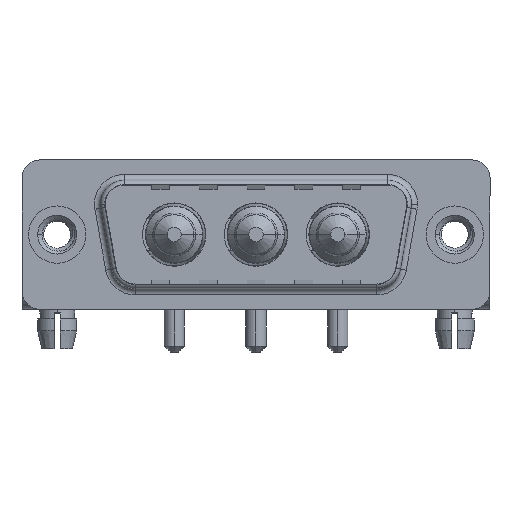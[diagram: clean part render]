
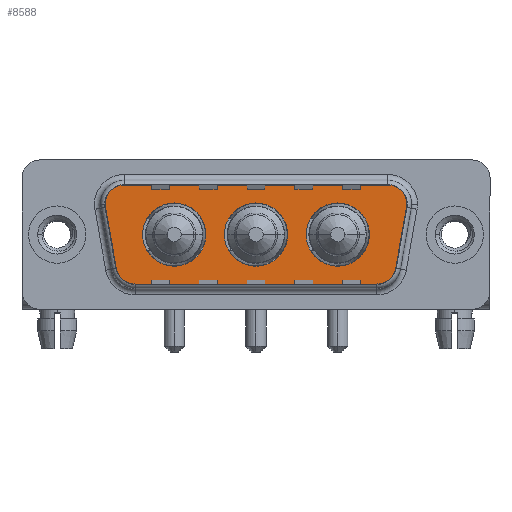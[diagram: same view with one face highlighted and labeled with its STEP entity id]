
A CAD part, top view. The second image highlights one B-rep face of the part: STEP entity #8588.
In plain terms, the highlighted planar face has unit normal (0, 0, 1).
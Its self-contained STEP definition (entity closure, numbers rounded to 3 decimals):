
#421 = ORIENTED_EDGE ( 'NONE', *, *, #2245, .F. ) ;
#662 = VERTEX_POINT ( 'NONE', #5880 ) ;
#727 = DIRECTION ( 'NONE',  ( 0.174, -0.985, 0. ) ) ;
#827 = DIRECTION ( 'NONE',  ( 0., 0., 1. ) ) ;
#843 = AXIS2_PLACEMENT_3D ( 'NONE', #4515, #4436, #9193 ) ;
#875 = EDGE_CURVE ( 'NONE', #9077, #4054, #5537, .T. ) ;
#971 = VECTOR ( 'NONE', #7393, 1000. ) ;
#1260 = CARTESIAN_POINT ( 'NONE',  ( 19.3, 0., 0. ) ) ;
#1284 = DIRECTION ( 'NONE',  ( 1., 0., 0. ) ) ;
#1347 = DIRECTION ( 'NONE',  ( 0., 0., 1. ) ) ;
#1507 = VECTOR ( 'NONE', #13732, 1000. ) ;
#1747 = VERTEX_POINT ( 'NONE', #15391 ) ;
#1857 = CARTESIAN_POINT ( 'NONE',  ( 26.866, -4.9, 0. ) ) ;
#1952 = ORIENTED_EDGE ( 'NONE', *, *, #10803, .F. ) ;
#2059 = CARTESIAN_POINT ( 'NONE',  ( 16.65, 0., 0. ) ) ;
#2143 = CARTESIAN_POINT ( 'NONE',  ( 3.441, 2.553, 0. ) ) ;
#2179 = AXIS2_PLACEMENT_3D ( 'NONE', #13234, #3705, #9710 ) ;
#2240 = CARTESIAN_POINT ( 'NONE',  ( 6.434, -4.9, 0. ) ) ;
#2245 = EDGE_CURVE ( 'NONE', #8454, #3330, #14317, .T. ) ;
#2381 = AXIS2_PLACEMENT_3D ( 'NONE', #6472, #11248, #10149 ) ;
#2434 = DIRECTION ( 'NONE',  ( 1., 0., 0. ) ) ;
#2448 = DIRECTION ( 'NONE',  ( 0., 0., 1. ) ) ;
#2454 = LINE ( 'NONE', #5647, #15405 ) ;
#2497 = EDGE_CURVE ( 'NONE', #8387, #662, #7977, .T. ) ;
#2549 = EDGE_CURVE ( 'NONE', #3667, #9077, #8069, .T. ) ;
#2558 = AXIS2_PLACEMENT_3D ( 'NONE', #6424, #7535, #4093 ) ;
#2796 = LINE ( 'NONE', #6372, #1507 ) ;
#2997 = VECTOR ( 'NONE', #727, 1000. ) ;
#3062 = EDGE_LOOP ( 'NONE', ( #7144, #14014, #3810, #6294, #6666, #3516, #14656, #10822, #7431 ) ) ;
#3122 = CARTESIAN_POINT ( 'NONE',  ( 29.859, 2.553, 0. ) ) ;
#3330 = VERTEX_POINT ( 'NONE', #1260 ) ;
#3516 = ORIENTED_EDGE ( 'NONE', *, *, #11779, .T. ) ;
#3667 = VERTEX_POINT ( 'NONE', #10840 ) ;
#3674 = CIRCLE ( 'NONE', #14910, 2.65 ) ;
#3705 = DIRECTION ( 'NONE',  ( 0., 0., 1. ) ) ;
#3810 = ORIENTED_EDGE ( 'NONE', *, *, #10605, .T. ) ;
#3811 = LINE ( 'NONE', #7470, #971 ) ;
#3848 = PLANE ( 'NONE',  #14581 ) ;
#3890 = EDGE_CURVE ( 'NONE', #1747, #4770, #2796, .T. ) ;
#3904 = AXIS2_PLACEMENT_3D ( 'NONE', #12129, #2448, #1284 ) ;
#3935 = ORIENTED_EDGE ( 'NONE', *, *, #12192, .F. ) ;
#4054 = VERTEX_POINT ( 'NONE', #2240 ) ;
#4093 = DIRECTION ( 'NONE',  ( -1., 0., 0. ) ) ;
#4250 = CARTESIAN_POINT ( 'NONE',  ( 26.866, -2.9, 0. ) ) ;
#4436 = DIRECTION ( 'NONE',  ( 0., 0., 1. ) ) ;
#4515 = CARTESIAN_POINT ( 'NONE',  ( 16.65, 0., 0. ) ) ;
#4540 = ORIENTED_EDGE ( 'NONE', *, *, #11421, .F. ) ;
#4614 = CIRCLE ( 'NONE', #2381, 2.65 ) ;
#4641 = EDGE_LOOP ( 'NONE', ( #4540, #5995 ) ) ;
#4712 = VERTEX_POINT ( 'NONE', #3122 ) ;
#4770 = VERTEX_POINT ( 'NONE', #7727 ) ;
#5025 = FACE_BOUND ( 'NONE', #14420, .T. ) ;
#5050 = VERTEX_POINT ( 'NONE', #6220 ) ;
#5155 = CARTESIAN_POINT ( 'NONE',  ( 4.464, -3.247, 0. ) ) ;
#5161 = CARTESIAN_POINT ( 'NONE',  ( 26.15, 0., 0. ) ) ;
#5177 = DIRECTION ( 'NONE',  ( 1., 0., 0. ) ) ;
#5186 = AXIS2_PLACEMENT_3D ( 'NONE', #14617, #1347, #2434 ) ;
#5260 = EDGE_LOOP ( 'NONE', ( #1952, #421 ) ) ;
#5520 = CARTESIAN_POINT ( 'NONE',  ( 29.889, 2.9, 0. ) ) ;
#5537 = CIRCLE ( 'NONE', #2558, 2. ) ;
#5647 = CARTESIAN_POINT ( 'NONE',  ( 29.859, 2.553, 0. ) ) ;
#5720 = AXIS2_PLACEMENT_3D ( 'NONE', #4250, #12600, #12753 ) ;
#5880 = CARTESIAN_POINT ( 'NONE',  ( 28.836, -3.247, 0. ) ) ;
#5995 = ORIENTED_EDGE ( 'NONE', *, *, #9329, .F. ) ;
#6144 = EDGE_CURVE ( 'NONE', #6786, #5050, #11372, .T. ) ;
#6185 = DIRECTION ( 'NONE',  ( 0., 0., 1. ) ) ;
#6220 = CARTESIAN_POINT ( 'NONE',  ( 12.45, 0., 0. ) ) ;
#6294 = ORIENTED_EDGE ( 'NONE', *, *, #6373, .T. ) ;
#6372 = CARTESIAN_POINT ( 'NONE',  ( 5.411, 4.9, 0. ) ) ;
#6373 = EDGE_CURVE ( 'NONE', #6789, #1747, #10601, .T. ) ;
#6424 = CARTESIAN_POINT ( 'NONE',  ( 6.434, -2.9, 0. ) ) ;
#6472 = CARTESIAN_POINT ( 'NONE',  ( 23.5, 0., 0. ) ) ;
#6666 = ORIENTED_EDGE ( 'NONE', *, *, #3890, .T. ) ;
#6786 = VERTEX_POINT ( 'NONE', #11460 ) ;
#6789 = VERTEX_POINT ( 'NONE', #5520 ) ;
#7144 = ORIENTED_EDGE ( 'NONE', *, *, #2497, .T. ) ;
#7393 = DIRECTION ( 'NONE',  ( 1., 0., 0. ) ) ;
#7431 = ORIENTED_EDGE ( 'NONE', *, *, #14473, .T. ) ;
#7470 = CARTESIAN_POINT ( 'NONE',  ( 6.434, -4.9, 0. ) ) ;
#7535 = DIRECTION ( 'NONE',  ( 0., 0., 1. ) ) ;
#7597 = FACE_BOUND ( 'NONE', #4641, .T. ) ;
#7727 = CARTESIAN_POINT ( 'NONE',  ( 5.411, 4.9, 0. ) ) ;
#7897 = DIRECTION ( 'NONE',  ( 0., 0., 1. ) ) ;
#7977 = CIRCLE ( 'NONE', #5720, 2. ) ;
#8069 = LINE ( 'NONE', #2143, #2997 ) ;
#8387 = VERTEX_POINT ( 'NONE', #1857 ) ;
#8428 = CIRCLE ( 'NONE', #5186, 2.65 ) ;
#8454 = VERTEX_POINT ( 'NONE', #10804 ) ;
#8588 = ADVANCED_FACE ( 'NONE', ( #12357, #7597, #5025, #13457 ), #3848, .T. ) ;
#8621 = VERTEX_POINT ( 'NONE', #9702 ) ;
#8667 = CIRCLE ( 'NONE', #11404, 2. ) ;
#9077 = VERTEX_POINT ( 'NONE', #5155 ) ;
#9193 = DIRECTION ( 'NONE',  ( 1., 0., 0. ) ) ;
#9305 = DIRECTION ( 'NONE',  ( 1., 0., 0. ) ) ;
#9329 = EDGE_CURVE ( 'NONE', #8621, #13535, #4614, .T. ) ;
#9382 = CIRCLE ( 'NONE', #2179, 2. ) ;
#9702 = CARTESIAN_POINT ( 'NONE',  ( 20.85, 0., 0. ) ) ;
#9710 = DIRECTION ( 'NONE',  ( -1., 0., 0. ) ) ;
#9884 = CIRCLE ( 'NONE', #12886, 2.65 ) ;
#10149 = DIRECTION ( 'NONE',  ( 1., 0., 0. ) ) ;
#10170 = DIRECTION ( 'NONE',  ( -1., 0., 0. ) ) ;
#10601 = CIRCLE ( 'NONE', #14594, 2. ) ;
#10605 = EDGE_CURVE ( 'NONE', #4712, #6789, #9382, .T. ) ;
#10803 = EDGE_CURVE ( 'NONE', #3330, #8454, #9884, .T. ) ;
#10804 = CARTESIAN_POINT ( 'NONE',  ( 14., 0., 0. ) ) ;
#10814 = DIRECTION ( 'NONE',  ( 0.174, 0.985, 0. ) ) ;
#10822 = ORIENTED_EDGE ( 'NONE', *, *, #875, .T. ) ;
#10840 = CARTESIAN_POINT ( 'NONE',  ( 3.441, 2.553, 0. ) ) ;
#10956 = DIRECTION ( 'NONE',  ( 0., 0., 1. ) ) ;
#11248 = DIRECTION ( 'NONE',  ( 0., 0., 1. ) ) ;
#11372 = CIRCLE ( 'NONE', #3904, 2.65 ) ;
#11404 = AXIS2_PLACEMENT_3D ( 'NONE', #12061, #6185, #5177 ) ;
#11421 = EDGE_CURVE ( 'NONE', #13535, #8621, #3674, .T. ) ;
#11460 = CARTESIAN_POINT ( 'NONE',  ( 7.15, 0., 0. ) ) ;
#11684 = EDGE_CURVE ( 'NONE', #662, #4712, #2454, .T. ) ;
#11779 = EDGE_CURVE ( 'NONE', #4770, #3667, #8667, .T. ) ;
#12061 = CARTESIAN_POINT ( 'NONE',  ( 5.411, 2.9, 0. ) ) ;
#12129 = CARTESIAN_POINT ( 'NONE',  ( 9.8, 0., 0. ) ) ;
#12192 = EDGE_CURVE ( 'NONE', #5050, #6786, #8428, .T. ) ;
#12282 = DIRECTION ( 'NONE',  ( 1., 0., 0. ) ) ;
#12357 = FACE_BOUND ( 'NONE', #5260, .T. ) ;
#12536 = DIRECTION ( 'NONE',  ( 1., 0., 0. ) ) ;
#12600 = DIRECTION ( 'NONE',  ( 0., 0., 1. ) ) ;
#12753 = DIRECTION ( 'NONE',  ( 1., 0., 0. ) ) ;
#12817 = DIRECTION ( 'NONE',  ( 0., 0., 1. ) ) ;
#12886 = AXIS2_PLACEMENT_3D ( 'NONE', #2059, #12817, #9305 ) ;
#13234 = CARTESIAN_POINT ( 'NONE',  ( 27.889, 2.9, 0. ) ) ;
#13457 = FACE_OUTER_BOUND ( 'NONE', #3062, .T. ) ;
#13535 = VERTEX_POINT ( 'NONE', #5161 ) ;
#13543 = CARTESIAN_POINT ( 'NONE',  ( 26.866, -2.9, 0. ) ) ;
#13644 = CARTESIAN_POINT ( 'NONE',  ( 23.5, 0., 0. ) ) ;
#13732 = DIRECTION ( 'NONE',  ( -1., 0., 0. ) ) ;
#14014 = ORIENTED_EDGE ( 'NONE', *, *, #11684, .T. ) ;
#14137 = CARTESIAN_POINT ( 'NONE',  ( 27.889, 2.9, 0. ) ) ;
#14317 = CIRCLE ( 'NONE', #843, 2.65 ) ;
#14420 = EDGE_LOOP ( 'NONE', ( #3935, #14726 ) ) ;
#14473 = EDGE_CURVE ( 'NONE', #4054, #8387, #3811, .T. ) ;
#14581 = AXIS2_PLACEMENT_3D ( 'NONE', #13543, #10956, #12282 ) ;
#14594 = AXIS2_PLACEMENT_3D ( 'NONE', #14137, #7897, #10170 ) ;
#14617 = CARTESIAN_POINT ( 'NONE',  ( 9.8, 0., 0. ) ) ;
#14656 = ORIENTED_EDGE ( 'NONE', *, *, #2549, .T. ) ;
#14726 = ORIENTED_EDGE ( 'NONE', *, *, #6144, .F. ) ;
#14910 = AXIS2_PLACEMENT_3D ( 'NONE', #13644, #827, #12536 ) ;
#15391 = CARTESIAN_POINT ( 'NONE',  ( 27.889, 4.9, 0. ) ) ;
#15405 = VECTOR ( 'NONE', #10814, 1000. ) ;
